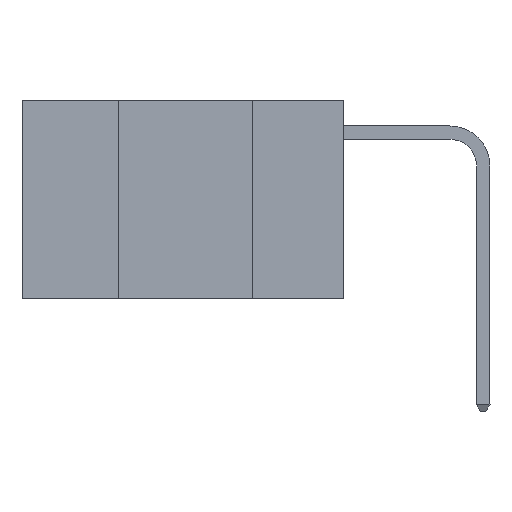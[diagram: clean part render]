
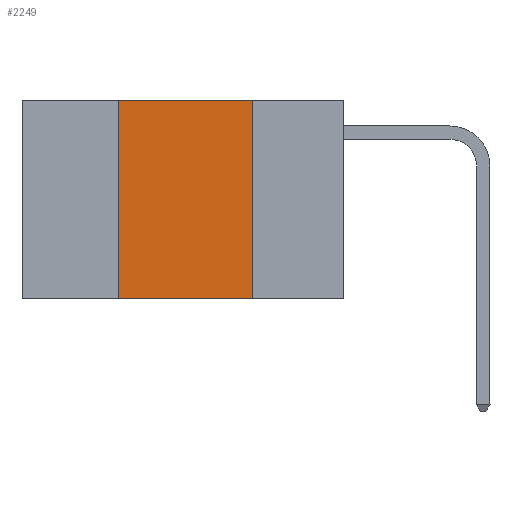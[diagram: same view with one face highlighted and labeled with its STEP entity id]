
A CAD part, left-side view. The second image highlights one B-rep face of the part: STEP entity #2249.
In plain terms, the highlighted planar face has unit normal (-1, 0, 0).
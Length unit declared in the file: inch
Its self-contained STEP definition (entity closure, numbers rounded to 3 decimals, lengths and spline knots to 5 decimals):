
#257 = DIRECTION ( 'NONE',  ( 1., 0., 0. ) ) ;
#1612 = DIRECTION ( 'NONE',  ( 0., 0., -1. ) ) ;
#1764 = FACE_OUTER_BOUND ( 'NONE', #1833, .T. ) ;
#1833 = EDGE_LOOP ( 'NONE', ( #13238, #8446, #10135, #4008 ) ) ;
#2215 = LINE ( 'NONE', #6876, #5067 ) ;
#2249 = ADVANCED_FACE ( 'NONE', ( #1764 ), #2335, .F. ) ;
#2334 = VERTEX_POINT ( 'NONE', #12935 ) ;
#2335 = PLANE ( 'NONE',  #5334 ) ;
#3248 = DIRECTION ( 'NONE',  ( 0., -1., 0. ) ) ;
#4008 = ORIENTED_EDGE ( 'NONE', *, *, #13743, .T. ) ;
#4715 = DIRECTION ( 'NONE',  ( 0., 0., -1. ) ) ;
#5067 = VECTOR ( 'NONE', #3248, 39.37008 ) ;
#5113 = VECTOR ( 'NONE', #1612, 39.37008 ) ;
#5334 = AXIS2_PLACEMENT_3D ( 'NONE', #7074, #257, #4715 ) ;
#5447 = LINE ( 'NONE', #11311, #11535 ) ;
#5459 = DIRECTION ( 'NONE',  ( 0., 0., 1. ) ) ;
#5510 = EDGE_CURVE ( 'NONE', #12103, #14495, #9694, .T. ) ;
#5529 = CARTESIAN_POINT ( 'NONE',  ( 0., 0.42, 0. ) ) ;
#5576 = EDGE_CURVE ( 'NONE', #7747, #2334, #14422, .T. ) ;
#6803 = CARTESIAN_POINT ( 'NONE',  ( 0., 0.17, 0. ) ) ;
#6876 = CARTESIAN_POINT ( 'NONE',  ( 0., 0.6, -0.37 ) ) ;
#6992 = CARTESIAN_POINT ( 'NONE',  ( 0., 0.42, -0.37 ) ) ;
#7074 = CARTESIAN_POINT ( 'NONE',  ( 0., 0.6, 0. ) ) ;
#7363 = CARTESIAN_POINT ( 'NONE',  ( 0., 0.17, -0.37 ) ) ;
#7747 = VERTEX_POINT ( 'NONE', #6992 ) ;
#8446 = ORIENTED_EDGE ( 'NONE', *, *, #12960, .F. ) ;
#9694 = LINE ( 'NONE', #11913, #5113 ) ;
#10135 = ORIENTED_EDGE ( 'NONE', *, *, #5576, .F. ) ;
#11261 = VECTOR ( 'NONE', #5459, 39.37008 ) ;
#11311 = CARTESIAN_POINT ( 'NONE',  ( 0., 0.6, 0. ) ) ;
#11535 = VECTOR ( 'NONE', #13369, 39.37008 ) ;
#11913 = CARTESIAN_POINT ( 'NONE',  ( 0., 0.17, 0. ) ) ;
#12103 = VERTEX_POINT ( 'NONE', #6803 ) ;
#12935 = CARTESIAN_POINT ( 'NONE',  ( 0., 0.42, 0. ) ) ;
#12960 = EDGE_CURVE ( 'NONE', #2334, #12103, #5447, .T. ) ;
#13238 = ORIENTED_EDGE ( 'NONE', *, *, #5510, .F. ) ;
#13369 = DIRECTION ( 'NONE',  ( 0., -1., 0. ) ) ;
#13743 = EDGE_CURVE ( 'NONE', #7747, #14495, #2215, .T. ) ;
#14422 = LINE ( 'NONE', #5529, #11261 ) ;
#14495 = VERTEX_POINT ( 'NONE', #7363 ) ;
